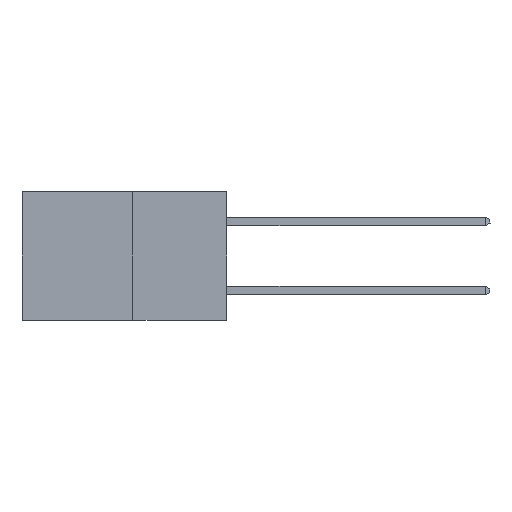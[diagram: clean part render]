
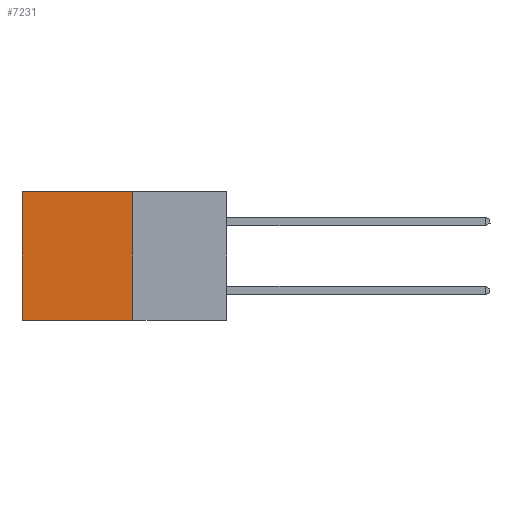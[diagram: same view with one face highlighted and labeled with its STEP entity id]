
A CAD part, left-side view. The second image highlights one B-rep face of the part: STEP entity #7231.
In plain terms, the highlighted planar face has unit normal (-1, 0, 0).
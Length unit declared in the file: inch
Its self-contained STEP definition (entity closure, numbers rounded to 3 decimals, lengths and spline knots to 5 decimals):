
#406 = VECTOR ( 'NONE', #9086, 39.37008 ) ;
#686 = EDGE_CURVE ( 'NONE', #5922, #8303, #3508, .T. ) ;
#1496 = VECTOR ( 'NONE', #2099, 39.37008 ) ;
#1598 = CARTESIAN_POINT ( 'NONE',  ( 0.277, 0.27, -0.37 ) ) ;
#2062 = VECTOR ( 'NONE', #12220, 39.37008 ) ;
#2099 = DIRECTION ( 'NONE',  ( 0., 0., -1. ) ) ;
#2292 = ORIENTED_EDGE ( 'NONE', *, *, #686, .F. ) ;
#2404 = EDGE_CURVE ( 'NONE', #5082, #5922, #12423, .T. ) ;
#2832 = CARTESIAN_POINT ( 'NONE',  ( 0.277, 0.59, 0. ) ) ;
#2974 = CARTESIAN_POINT ( 'NONE',  ( 0.277, 0.27, 0. ) ) ;
#3508 = LINE ( 'NONE', #6982, #406 ) ;
#3809 = PLANE ( 'NONE',  #9678 ) ;
#4828 = DIRECTION ( 'NONE',  ( 0., 0., -1. ) ) ;
#5082 = VERTEX_POINT ( 'NONE', #12466 ) ;
#5922 = VERTEX_POINT ( 'NONE', #10766 ) ;
#6816 = EDGE_CURVE ( 'NONE', #11494, #8303, #11056, .T. ) ;
#6982 = CARTESIAN_POINT ( 'NONE',  ( 0.277, 0.27, -0.37 ) ) ;
#7231 = ADVANCED_FACE ( 'NONE', ( #7512 ), #3809, .F. ) ;
#7351 = LINE ( 'NONE', #2974, #12064 ) ;
#7512 = FACE_OUTER_BOUND ( 'NONE', #10940, .T. ) ;
#7884 = ORIENTED_EDGE ( 'NONE', *, *, #2404, .F. ) ;
#8182 = ORIENTED_EDGE ( 'NONE', *, *, #12904, .T. ) ;
#8303 = VERTEX_POINT ( 'NONE', #9762 ) ;
#9086 = DIRECTION ( 'NONE',  ( 0., 1., 0. ) ) ;
#9678 = AXIS2_PLACEMENT_3D ( 'NONE', #1598, #10501, #4828 ) ;
#9738 = DIRECTION ( 'NONE',  ( 0., 1., 0. ) ) ;
#9762 = CARTESIAN_POINT ( 'NONE',  ( 0.277, 0.59, -0.37 ) ) ;
#9947 = CARTESIAN_POINT ( 'NONE',  ( 0.277, 0.59, -0.37 ) ) ;
#10501 = DIRECTION ( 'NONE',  ( 1., 0., 0. ) ) ;
#10766 = CARTESIAN_POINT ( 'NONE',  ( 0.277, 0.27, -0.37 ) ) ;
#10940 = EDGE_LOOP ( 'NONE', ( #12008, #2292, #7884, #8182 ) ) ;
#11056 = LINE ( 'NONE', #9947, #1496 ) ;
#11494 = VERTEX_POINT ( 'NONE', #2832 ) ;
#11958 = CARTESIAN_POINT ( 'NONE',  ( 0.277, 0.27, -0.37 ) ) ;
#12008 = ORIENTED_EDGE ( 'NONE', *, *, #6816, .T. ) ;
#12064 = VECTOR ( 'NONE', #9738, 39.37008 ) ;
#12220 = DIRECTION ( 'NONE',  ( 0., 0., -1. ) ) ;
#12423 = LINE ( 'NONE', #11958, #2062 ) ;
#12466 = CARTESIAN_POINT ( 'NONE',  ( 0.277, 0.27, 0. ) ) ;
#12904 = EDGE_CURVE ( 'NONE', #5082, #11494, #7351, .T. ) ;
